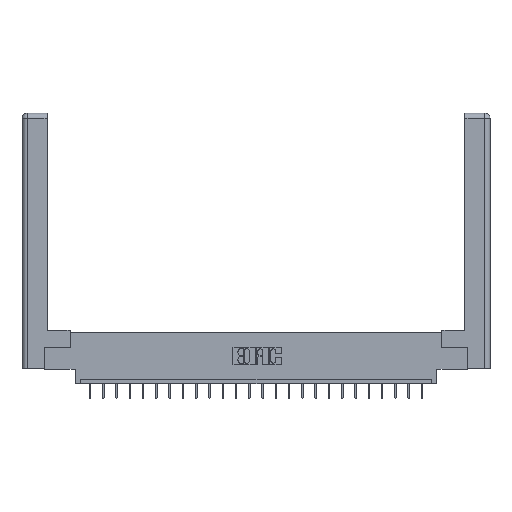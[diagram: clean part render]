
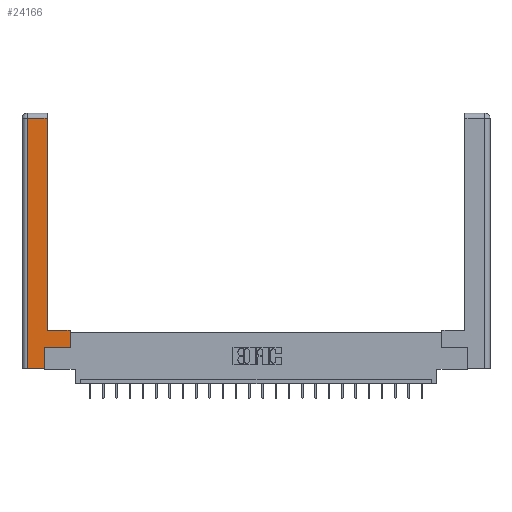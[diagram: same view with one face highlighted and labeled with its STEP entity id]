
A CAD part, top view. The second image highlights one B-rep face of the part: STEP entity #24166.
In plain terms, the highlighted planar face has unit normal (0, 0, 1).
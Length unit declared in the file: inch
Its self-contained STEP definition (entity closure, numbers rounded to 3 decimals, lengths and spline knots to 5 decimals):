
#543 = CARTESIAN_POINT ( 'NONE',  ( 0.265, 0., 0. ) ) ;
#964 = LINE ( 'NONE', #11103, #2156 ) ;
#1227 = AXIS2_PLACEMENT_3D ( 'NONE', #22234, #1569, #1736 ) ;
#1397 = VERTEX_POINT ( 'NONE', #16653 ) ;
#1569 = DIRECTION ( 'NONE',  ( 0., 0., -1. ) ) ;
#1736 = DIRECTION ( 'NONE',  ( -1., 0., 0. ) ) ;
#2067 = DIRECTION ( 'NONE',  ( 0., 1., 0. ) ) ;
#2142 = CARTESIAN_POINT ( 'NONE',  ( 0.295, 3., 0. ) ) ;
#2156 = VECTOR ( 'NONE', #14892, 39.37008 ) ;
#2420 = VERTEX_POINT ( 'NONE', #9720 ) ;
#2519 = ORIENTED_EDGE ( 'NONE', *, *, #23300, .T. ) ;
#2542 = VECTOR ( 'NONE', #7901, 39.37008 ) ;
#3593 = VERTEX_POINT ( 'NONE', #12194 ) ;
#5984 = DIRECTION ( 'NONE',  ( -1., 0., 0. ) ) ;
#6010 = CARTESIAN_POINT ( 'NONE',  ( 0.265, 0., 0. ) ) ;
#6450 = LINE ( 'NONE', #9732, #7929 ) ;
#6544 = VERTEX_POINT ( 'NONE', #11650 ) ;
#6750 = LINE ( 'NONE', #9943, #16124 ) ;
#6766 = LINE ( 'NONE', #543, #17598 ) ;
#7901 = DIRECTION ( 'NONE',  ( 1., 0., 0. ) ) ;
#7929 = VECTOR ( 'NONE', #5984, 39.37008 ) ;
#8097 = LINE ( 'NONE', #11553, #2542 ) ;
#8582 = CARTESIAN_POINT ( 'NONE',  ( 0.0615, 2.94, 0. ) ) ;
#8879 = ORIENTED_EDGE ( 'NONE', *, *, #14264, .T. ) ;
#8897 = EDGE_CURVE ( 'NONE', #6544, #13282, #964, .T. ) ;
#9606 = DIRECTION ( 'NONE',  ( 0., 1., 0. ) ) ;
#9720 = CARTESIAN_POINT ( 'NONE',  ( 0.295, 0.45, 0. ) ) ;
#9732 = CARTESIAN_POINT ( 'NONE',  ( 0.295, 0.45, 0. ) ) ;
#9943 = CARTESIAN_POINT ( 'NONE',  ( 0.565, 0.45, 0. ) ) ;
#10455 = ORIENTED_EDGE ( 'NONE', *, *, #19903, .T. ) ;
#10785 = EDGE_CURVE ( 'NONE', #1397, #6544, #21965, .T. ) ;
#11000 = EDGE_LOOP ( 'NONE', ( #8879, #16315, #23108, #17158, #10455, #2519, #11800, #23400 ) ) ;
#11026 = EDGE_CURVE ( 'NONE', #3593, #2420, #6450, .T. ) ;
#11103 = CARTESIAN_POINT ( 'NONE',  ( 0.0615, 0., 0. ) ) ;
#11405 = CARTESIAN_POINT ( 'NONE',  ( 0.0615, 0., 0. ) ) ;
#11553 = CARTESIAN_POINT ( 'NONE',  ( 0.565, 0.245, 0. ) ) ;
#11650 = CARTESIAN_POINT ( 'NONE',  ( 0.0615, 2.94, 0. ) ) ;
#11800 = ORIENTED_EDGE ( 'NONE', *, *, #18830, .T. ) ;
#11822 = DIRECTION ( 'NONE',  ( 1., 0., 0. ) ) ;
#12178 = VERTEX_POINT ( 'NONE', #21502 ) ;
#12194 = CARTESIAN_POINT ( 'NONE',  ( 0.565, 0.45, 0. ) ) ;
#12768 = PLANE ( 'NONE',  #1227 ) ;
#13282 = VERTEX_POINT ( 'NONE', #11405 ) ;
#13285 = VERTEX_POINT ( 'NONE', #22275 ) ;
#13592 = VERTEX_POINT ( 'NONE', #6010 ) ;
#14018 = VECTOR ( 'NONE', #9606, 39.37008 ) ;
#14264 = EDGE_CURVE ( 'NONE', #2420, #1397, #21324, .T. ) ;
#14892 = DIRECTION ( 'NONE',  ( 0., -1., 0. ) ) ;
#14967 = VECTOR ( 'NONE', #21370, 39.37008 ) ;
#16124 = VECTOR ( 'NONE', #17453, 39.37008 ) ;
#16315 = ORIENTED_EDGE ( 'NONE', *, *, #10785, .T. ) ;
#16653 = CARTESIAN_POINT ( 'NONE',  ( 0.295, 2.94, 0. ) ) ;
#17158 = ORIENTED_EDGE ( 'NONE', *, *, #17651, .T. ) ;
#17453 = DIRECTION ( 'NONE',  ( 0., 1., 0. ) ) ;
#17598 = VECTOR ( 'NONE', #11822, 39.37008 ) ;
#17651 = EDGE_CURVE ( 'NONE', #13282, #13592, #6766, .T. ) ;
#17804 = LINE ( 'NONE', #18952, #14018 ) ;
#18830 = EDGE_CURVE ( 'NONE', #13285, #3593, #6750, .T. ) ;
#18952 = CARTESIAN_POINT ( 'NONE',  ( 0.265, 0.245, 0. ) ) ;
#19903 = EDGE_CURVE ( 'NONE', #13592, #12178, #17804, .T. ) ;
#21324 = LINE ( 'NONE', #2142, #22773 ) ;
#21370 = DIRECTION ( 'NONE',  ( -1., 0., 0. ) ) ;
#21502 = CARTESIAN_POINT ( 'NONE',  ( 0.265, 0.245, 0. ) ) ;
#21786 = FACE_OUTER_BOUND ( 'NONE', #11000, .T. ) ;
#21965 = LINE ( 'NONE', #8582, #14967 ) ;
#22234 = CARTESIAN_POINT ( 'NONE',  ( 0., 0., 0. ) ) ;
#22275 = CARTESIAN_POINT ( 'NONE',  ( 0.565, 0.245, 0. ) ) ;
#22773 = VECTOR ( 'NONE', #2067, 39.37008 ) ;
#23108 = ORIENTED_EDGE ( 'NONE', *, *, #8897, .T. ) ;
#23300 = EDGE_CURVE ( 'NONE', #12178, #13285, #8097, .T. ) ;
#23400 = ORIENTED_EDGE ( 'NONE', *, *, #11026, .T. ) ;
#24166 = ADVANCED_FACE ( 'NONE', ( #21786 ), #12768, .F. ) ;
